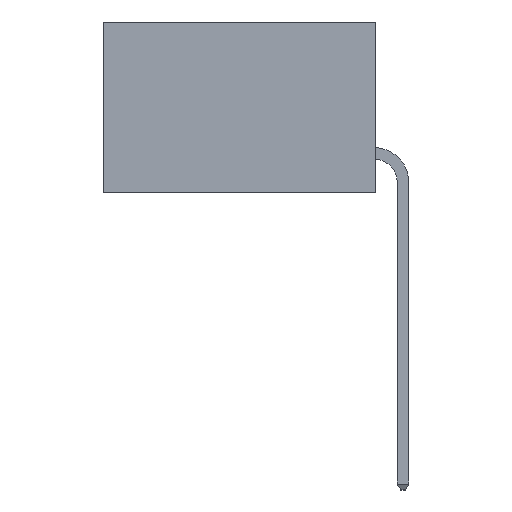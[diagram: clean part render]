
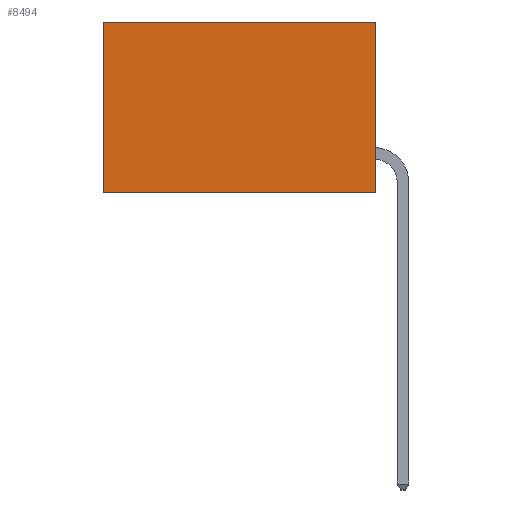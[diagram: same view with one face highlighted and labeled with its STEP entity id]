
A CAD part, left-side view. The second image highlights one B-rep face of the part: STEP entity #8494.
In plain terms, the highlighted planar face has unit normal (-1, 0, 0).
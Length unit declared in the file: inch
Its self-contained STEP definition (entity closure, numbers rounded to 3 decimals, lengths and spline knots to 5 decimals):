
#1100 = CARTESIAN_POINT ( 'NONE',  ( 0.277, 0.59, -0.37 ) ) ;
#1409 = CARTESIAN_POINT ( 'NONE',  ( 0.277, 0.59, 0. ) ) ;
#1565 = AXIS2_PLACEMENT_3D ( 'NONE', #15804, #5044, #17516 ) ;
#1667 = LINE ( 'NONE', #9257, #10806 ) ;
#2449 = EDGE_CURVE ( 'NONE', #3335, #6387, #11342, .T. ) ;
#2723 = DIRECTION ( 'NONE',  ( 0., 0., -1. ) ) ;
#2811 = VERTEX_POINT ( 'NONE', #1409 ) ;
#3196 = PLANE ( 'NONE',  #1565 ) ;
#3335 = VERTEX_POINT ( 'NONE', #9140 ) ;
#4464 = EDGE_LOOP ( 'NONE', ( #4782, #19979, #16578, #12411 ) ) ;
#4782 = ORIENTED_EDGE ( 'NONE', *, *, #20155, .T. ) ;
#5005 = EDGE_CURVE ( 'NONE', #6387, #9630, #6598, .T. ) ;
#5044 = DIRECTION ( 'NONE',  ( 1., 0., 0. ) ) ;
#6387 = VERTEX_POINT ( 'NONE', #11398 ) ;
#6598 = LINE ( 'NONE', #19476, #20079 ) ;
#7434 = DIRECTION ( 'NONE',  ( 0., 1., 0. ) ) ;
#8494 = ADVANCED_FACE ( 'NONE', ( #20288 ), #3196, .F. ) ;
#9140 = CARTESIAN_POINT ( 'NONE',  ( 0.277, 0., 0. ) ) ;
#9257 = CARTESIAN_POINT ( 'NONE',  ( 0.277, 0., 0. ) ) ;
#9630 = VERTEX_POINT ( 'NONE', #1100 ) ;
#10806 = VECTOR ( 'NONE', #7434, 39.37008 ) ;
#11342 = LINE ( 'NONE', #15644, #20027 ) ;
#11398 = CARTESIAN_POINT ( 'NONE',  ( 0.277, 0., -0.37 ) ) ;
#12411 = ORIENTED_EDGE ( 'NONE', *, *, #22637, .T. ) ;
#13582 = CARTESIAN_POINT ( 'NONE',  ( 0.277, 0.59, -0.37 ) ) ;
#15644 = CARTESIAN_POINT ( 'NONE',  ( 0.277, 0., -0.37 ) ) ;
#15804 = CARTESIAN_POINT ( 'NONE',  ( 0.277, 0., -0.37 ) ) ;
#16578 = ORIENTED_EDGE ( 'NONE', *, *, #2449, .F. ) ;
#17371 = DIRECTION ( 'NONE',  ( 0., 0., -1. ) ) ;
#17516 = DIRECTION ( 'NONE',  ( 0., 0., -1. ) ) ;
#19476 = CARTESIAN_POINT ( 'NONE',  ( 0.277, 0., -0.37 ) ) ;
#19480 = DIRECTION ( 'NONE',  ( 0., 1., 0. ) ) ;
#19979 = ORIENTED_EDGE ( 'NONE', *, *, #5005, .F. ) ;
#20027 = VECTOR ( 'NONE', #17371, 39.37008 ) ;
#20079 = VECTOR ( 'NONE', #19480, 39.37008 ) ;
#20155 = EDGE_CURVE ( 'NONE', #2811, #9630, #20920, .T. ) ;
#20288 = FACE_OUTER_BOUND ( 'NONE', #4464, .T. ) ;
#20920 = LINE ( 'NONE', #13582, #21448 ) ;
#21448 = VECTOR ( 'NONE', #2723, 39.37008 ) ;
#22637 = EDGE_CURVE ( 'NONE', #3335, #2811, #1667, .T. ) ;
